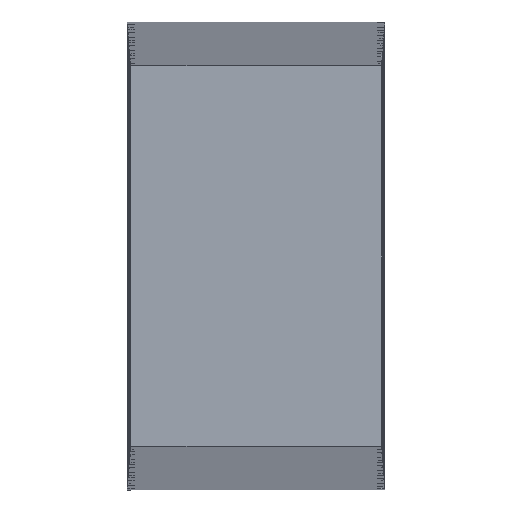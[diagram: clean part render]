
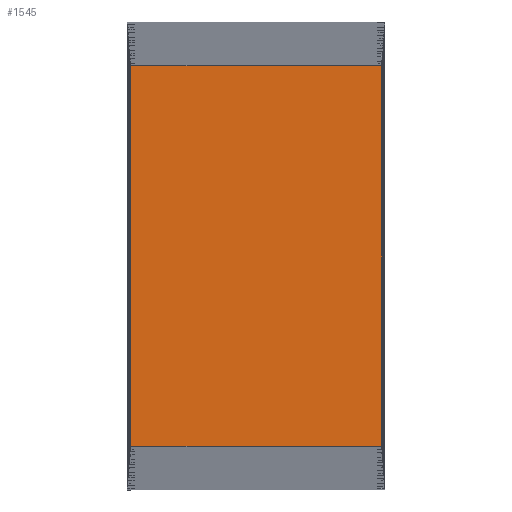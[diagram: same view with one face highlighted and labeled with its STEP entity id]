
A CAD part, front view. The second image highlights one B-rep face of the part: STEP entity #1545.
In plain terms, the highlighted planar face has unit normal (0, -1, 0).
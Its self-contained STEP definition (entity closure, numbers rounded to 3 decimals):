
#64=FACE_OUTER_BOUND('',#145,.T.);
#145=EDGE_LOOP('',(#1115,#1116,#1117,#1118));
#246=LINE('',#2229,#395);
#277=LINE('',#2384,#426);
#279=LINE('',#2388,#428);
#280=LINE('',#2389,#429);
#395=VECTOR('',#1814,10.);
#426=VECTOR('',#1897,10.);
#428=VECTOR('',#1901,10.);
#429=VECTOR('',#1902,10.);
#642=VERTEX_POINT('',#2226);
#643=VERTEX_POINT('',#2228);
#693=VERTEX_POINT('',#2383);
#694=VERTEX_POINT('',#2387);
#804=EDGE_CURVE('',#643,#642,#246,.T.);
#860=EDGE_CURVE('',#693,#643,#277,.T.);
#862=EDGE_CURVE('',#642,#694,#279,.T.);
#863=EDGE_CURVE('',#694,#693,#280,.T.);
#1115=ORIENTED_EDGE('',*,*,#804,.T.);
#1116=ORIENTED_EDGE('',*,*,#862,.T.);
#1117=ORIENTED_EDGE('',*,*,#863,.T.);
#1118=ORIENTED_EDGE('',*,*,#860,.T.);
#1503=PLANE('',#1682);
#1545=ADVANCED_FACE('',(#64),#1503,.F.);
#1682=AXIS2_PLACEMENT_3D('',#2386,#1899,#1900);
#1814=DIRECTION('',(-1.,0.,0.));
#1897=DIRECTION('',(0.,0.,1.));
#1899=DIRECTION('center_axis',(0.,1.,0.));
#1900=DIRECTION('ref_axis',(0.,0.,1.));
#1901=DIRECTION('',(0.,0.,-1.));
#1902=DIRECTION('',(1.,0.,0.));
#2226=CARTESIAN_POINT('',(-19.261,-239.951,-29.838));
#2228=CARTESIAN_POINT('',(-6.092,-239.95,-29.838));
#2229=CARTESIAN_POINT('',(-17.622,-239.951,-29.838));
#2383=CARTESIAN_POINT('',(-6.092,-239.95,-49.838));
#2384=CARTESIAN_POINT('',(-6.092,-239.95,-52.126));
#2386=CARTESIAN_POINT('Origin',(-12.677,-239.95,-39.838));
#2387=CARTESIAN_POINT('',(-19.261,-239.951,-49.838));
#2388=CARTESIAN_POINT('',(-19.261,-239.951,-27.55));
#2389=CARTESIAN_POINT('',(-17.622,-239.951,-49.838));
